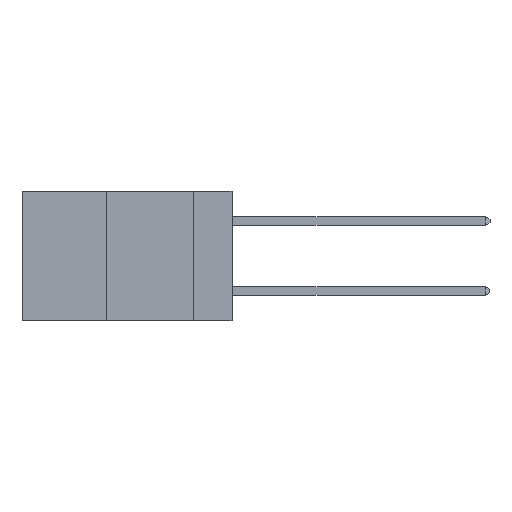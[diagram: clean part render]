
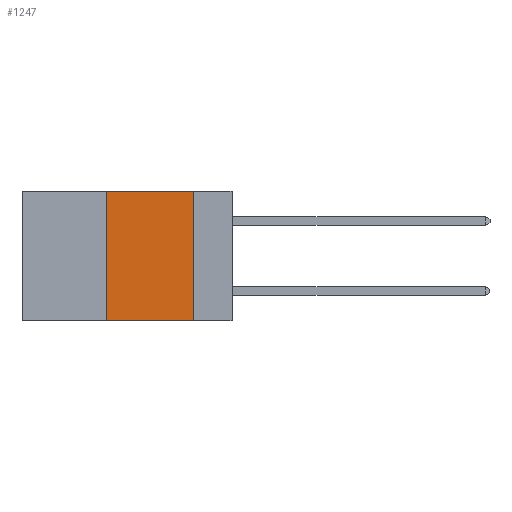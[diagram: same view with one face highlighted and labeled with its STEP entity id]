
A CAD part, left-side view. The second image highlights one B-rep face of the part: STEP entity #1247.
In plain terms, the highlighted planar face has unit normal (-1, 0, 0).
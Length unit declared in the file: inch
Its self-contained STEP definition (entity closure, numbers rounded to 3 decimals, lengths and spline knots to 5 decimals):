
#100 = VECTOR ( 'NONE', #5597, 39.37008 ) ;
#647 = EDGE_CURVE ( 'NONE', #5052, #6146, #10893, .T. ) ;
#851 = VECTOR ( 'NONE', #3399, 39.37008 ) ;
#1046 = EDGE_CURVE ( 'NONE', #2495, #5052, #11401, .T. ) ;
#1247 = ADVANCED_FACE ( 'NONE', ( #8151 ), #3290, .F. ) ;
#1654 = CARTESIAN_POINT ( 'NONE',  ( 0., 0.36, 0. ) ) ;
#2101 = VECTOR ( 'NONE', #4171, 39.37008 ) ;
#2211 = DIRECTION ( 'NONE',  ( 0., 0., -1. ) ) ;
#2314 = CARTESIAN_POINT ( 'NONE',  ( 0., 0.36, -0.37 ) ) ;
#2495 = VERTEX_POINT ( 'NONE', #2314 ) ;
#2644 = DIRECTION ( 'NONE',  ( 0., 0., -1. ) ) ;
#3126 = EDGE_CURVE ( 'NONE', #2495, #4798, #7974, .T. ) ;
#3290 = PLANE ( 'NONE',  #10520 ) ;
#3399 = DIRECTION ( 'NONE',  ( 0., -1., 0. ) ) ;
#3408 = CARTESIAN_POINT ( 'NONE',  ( 0., 0.6, 0. ) ) ;
#3512 = CARTESIAN_POINT ( 'NONE',  ( 0., 0.6, 0. ) ) ;
#4171 = DIRECTION ( 'NONE',  ( 0., 0., 1. ) ) ;
#4204 = CARTESIAN_POINT ( 'NONE',  ( 0., 0.11, 0. ) ) ;
#4400 = CARTESIAN_POINT ( 'NONE',  ( 0., 0.11, 0. ) ) ;
#4492 = DIRECTION ( 'NONE',  ( 1., 0., 0. ) ) ;
#4780 = CARTESIAN_POINT ( 'NONE',  ( 0., 0.11, -0.37 ) ) ;
#4798 = VERTEX_POINT ( 'NONE', #4780 ) ;
#5052 = VERTEX_POINT ( 'NONE', #8504 ) ;
#5597 = DIRECTION ( 'NONE',  ( 0., -1., 0. ) ) ;
#5699 = ORIENTED_EDGE ( 'NONE', *, *, #9965, .F. ) ;
#5916 = VECTOR ( 'NONE', #2644, 39.37008 ) ;
#6146 = VERTEX_POINT ( 'NONE', #4204 ) ;
#6287 = ORIENTED_EDGE ( 'NONE', *, *, #3126, .T. ) ;
#6844 = CARTESIAN_POINT ( 'NONE',  ( 0., 0.6, -0.37 ) ) ;
#7974 = LINE ( 'NONE', #6844, #851 ) ;
#8151 = FACE_OUTER_BOUND ( 'NONE', #9210, .T. ) ;
#8288 = LINE ( 'NONE', #4400, #5916 ) ;
#8504 = CARTESIAN_POINT ( 'NONE',  ( 0., 0.36, 0. ) ) ;
#8663 = ORIENTED_EDGE ( 'NONE', *, *, #647, .F. ) ;
#9210 = EDGE_LOOP ( 'NONE', ( #5699, #8663, #10158, #6287 ) ) ;
#9965 = EDGE_CURVE ( 'NONE', #6146, #4798, #8288, .T. ) ;
#10158 = ORIENTED_EDGE ( 'NONE', *, *, #1046, .F. ) ;
#10520 = AXIS2_PLACEMENT_3D ( 'NONE', #3408, #4492, #2211 ) ;
#10893 = LINE ( 'NONE', #3512, #100 ) ;
#11401 = LINE ( 'NONE', #1654, #2101 ) ;
